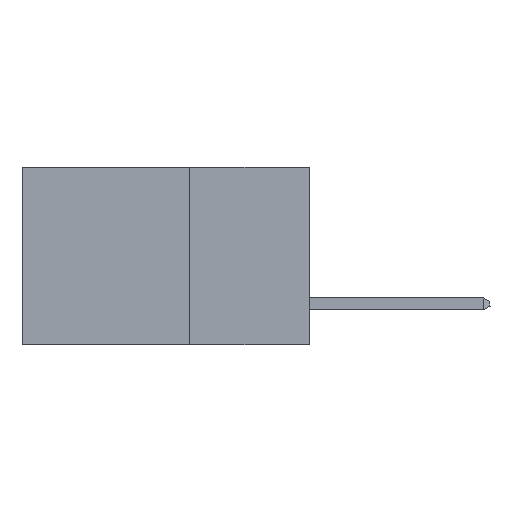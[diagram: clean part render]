
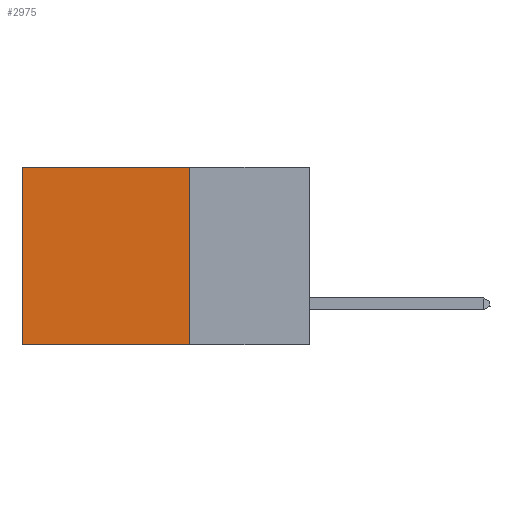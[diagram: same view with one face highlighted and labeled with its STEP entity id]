
A CAD part, left-side view. The second image highlights one B-rep face of the part: STEP entity #2975.
In plain terms, the highlighted planar face has unit normal (-1, 0, 0).
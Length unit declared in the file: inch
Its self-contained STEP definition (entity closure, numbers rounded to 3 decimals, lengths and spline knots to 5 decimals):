
#1148 = AXIS2_PLACEMENT_3D ( 'NONE', #10212, #6162, #18166 ) ;
#1741 = CARTESIAN_POINT ( 'NONE',  ( 0.2875, 0.6, 0. ) ) ;
#2588 = CARTESIAN_POINT ( 'NONE',  ( 0.2875, 0.25, 0. ) ) ;
#2975 = ADVANCED_FACE ( 'NONE', ( #23693 ), #21905, .F. ) ;
#3672 = DIRECTION ( 'NONE',  ( 0., 1., 0. ) ) ;
#3771 = EDGE_CURVE ( 'NONE', #24664, #8788, #9429, .T. ) ;
#5018 = ORIENTED_EDGE ( 'NONE', *, *, #3771, .T. ) ;
#5489 = CARTESIAN_POINT ( 'NONE',  ( 0.2875, 0.25, -0.37 ) ) ;
#5924 = CARTESIAN_POINT ( 'NONE',  ( 0.2875, 0.25, -0.37 ) ) ;
#6162 = DIRECTION ( 'NONE',  ( 1., 0., 0. ) ) ;
#6686 = VECTOR ( 'NONE', #3672, 39.37008 ) ;
#7805 = ORIENTED_EDGE ( 'NONE', *, *, #17377, .F. ) ;
#8183 = VECTOR ( 'NONE', #17979, 39.37008 ) ;
#8788 = VERTEX_POINT ( 'NONE', #25324 ) ;
#9429 = LINE ( 'NONE', #2588, #8183 ) ;
#9526 = DIRECTION ( 'NONE',  ( 0., 0., -1. ) ) ;
#10212 = CARTESIAN_POINT ( 'NONE',  ( 0.2875, 0.25, 0. ) ) ;
#10411 = LINE ( 'NONE', #5489, #6686 ) ;
#10455 = VERTEX_POINT ( 'NONE', #11148 ) ;
#11083 = VECTOR ( 'NONE', #11800, 39.37008 ) ;
#11148 = CARTESIAN_POINT ( 'NONE',  ( 0.2875, 0.6, -0.37 ) ) ;
#11547 = CARTESIAN_POINT ( 'NONE',  ( 0.2875, 0.25, 0. ) ) ;
#11800 = DIRECTION ( 'NONE',  ( 0., 0., -1. ) ) ;
#11967 = CARTESIAN_POINT ( 'NONE',  ( 0.2875, 0.25, 0. ) ) ;
#13615 = EDGE_CURVE ( 'NONE', #8788, #10455, #18373, .T. ) ;
#16201 = VERTEX_POINT ( 'NONE', #5924 ) ;
#16393 = ORIENTED_EDGE ( 'NONE', *, *, #25093, .F. ) ;
#17377 = EDGE_CURVE ( 'NONE', #24664, #16201, #24547, .T. ) ;
#17979 = DIRECTION ( 'NONE',  ( 0., 1., 0. ) ) ;
#18166 = DIRECTION ( 'NONE',  ( 0., 0., -1. ) ) ;
#18373 = LINE ( 'NONE', #1741, #22031 ) ;
#18411 = EDGE_LOOP ( 'NONE', ( #22349, #16393, #7805, #5018 ) ) ;
#21905 = PLANE ( 'NONE',  #1148 ) ;
#22031 = VECTOR ( 'NONE', #9526, 39.37008 ) ;
#22349 = ORIENTED_EDGE ( 'NONE', *, *, #13615, .T. ) ;
#23693 = FACE_OUTER_BOUND ( 'NONE', #18411, .T. ) ;
#24547 = LINE ( 'NONE', #11547, #11083 ) ;
#24664 = VERTEX_POINT ( 'NONE', #11967 ) ;
#25093 = EDGE_CURVE ( 'NONE', #16201, #10455, #10411, .T. ) ;
#25324 = CARTESIAN_POINT ( 'NONE',  ( 0.2875, 0.6, 0. ) ) ;
